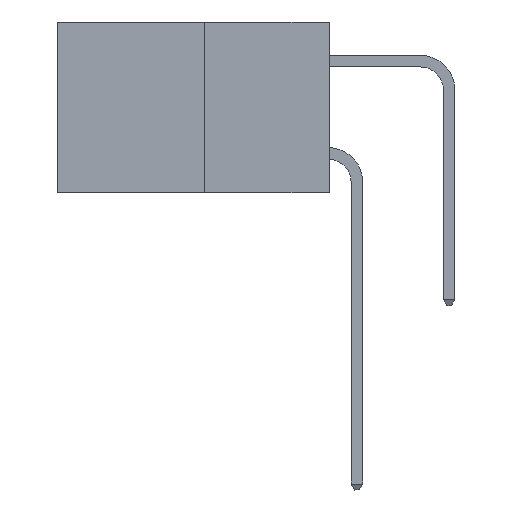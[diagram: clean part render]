
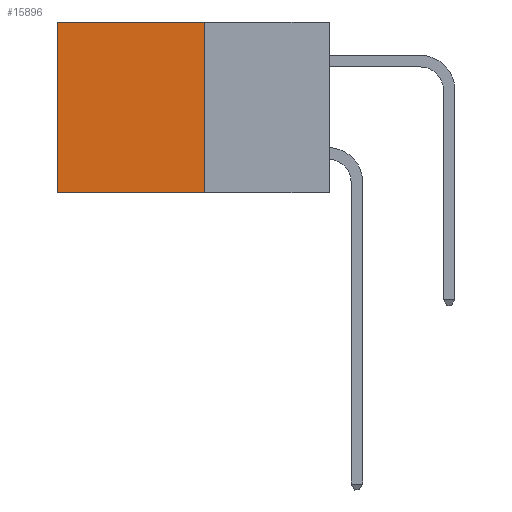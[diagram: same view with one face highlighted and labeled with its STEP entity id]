
A CAD part, left-side view. The second image highlights one B-rep face of the part: STEP entity #15896.
In plain terms, the highlighted planar face has unit normal (-1, 0, 0).
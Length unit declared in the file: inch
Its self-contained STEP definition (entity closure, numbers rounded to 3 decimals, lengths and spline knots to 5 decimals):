
#310 = CARTESIAN_POINT ( 'NONE',  ( 0.277, 0.27, -0.37 ) ) ;
#665 = LINE ( 'NONE', #18422, #26575 ) ;
#683 = FACE_OUTER_BOUND ( 'NONE', #27357, .T. ) ;
#1572 = LINE ( 'NONE', #18201, #24973 ) ;
#1852 = DIRECTION ( 'NONE',  ( 0., 1., 0. ) ) ;
#2089 = DIRECTION ( 'NONE',  ( 0., 0., -1. ) ) ;
#2840 = ORIENTED_EDGE ( 'NONE', *, *, #27835, .T. ) ;
#3052 = VECTOR ( 'NONE', #22208, 39.37008 ) ;
#5921 = CARTESIAN_POINT ( 'NONE',  ( 0.277, 0.59, 0. ) ) ;
#7754 = DIRECTION ( 'NONE',  ( 1., 0., 0. ) ) ;
#8976 = CARTESIAN_POINT ( 'NONE',  ( 0.277, 0.27, -0.37 ) ) ;
#10119 = EDGE_CURVE ( 'NONE', #29624, #12338, #15491, .T. ) ;
#10675 = ORIENTED_EDGE ( 'NONE', *, *, #14356, .T. ) ;
#12098 = LINE ( 'NONE', #27650, #23837 ) ;
#12338 = VERTEX_POINT ( 'NONE', #8976 ) ;
#13613 = EDGE_CURVE ( 'NONE', #12338, #26262, #1572, .T. ) ;
#14356 = EDGE_CURVE ( 'NONE', #29624, #16048, #12098, .T. ) ;
#14727 = CARTESIAN_POINT ( 'NONE',  ( 0.277, 0.27, -0.37 ) ) ;
#15491 = LINE ( 'NONE', #310, #3052 ) ;
#15896 = ADVANCED_FACE ( 'NONE', ( #683 ), #21793, .F. ) ;
#16048 = VERTEX_POINT ( 'NONE', #5921 ) ;
#18201 = CARTESIAN_POINT ( 'NONE',  ( 0.277, 0.27, -0.37 ) ) ;
#18422 = CARTESIAN_POINT ( 'NONE',  ( 0.277, 0.59, -0.37 ) ) ;
#21793 = PLANE ( 'NONE',  #25199 ) ;
#22208 = DIRECTION ( 'NONE',  ( 0., 0., -1. ) ) ;
#22405 = ORIENTED_EDGE ( 'NONE', *, *, #13613, .F. ) ;
#23837 = VECTOR ( 'NONE', #29986, 39.37008 ) ;
#24121 = DIRECTION ( 'NONE',  ( 0., 0., -1. ) ) ;
#24626 = ORIENTED_EDGE ( 'NONE', *, *, #10119, .F. ) ;
#24973 = VECTOR ( 'NONE', #1852, 39.37008 ) ;
#25199 = AXIS2_PLACEMENT_3D ( 'NONE', #14727, #7754, #24121 ) ;
#26055 = CARTESIAN_POINT ( 'NONE',  ( 0.277, 0.27, 0. ) ) ;
#26262 = VERTEX_POINT ( 'NONE', #26992 ) ;
#26575 = VECTOR ( 'NONE', #2089, 39.37008 ) ;
#26992 = CARTESIAN_POINT ( 'NONE',  ( 0.277, 0.59, -0.37 ) ) ;
#27357 = EDGE_LOOP ( 'NONE', ( #2840, #22405, #24626, #10675 ) ) ;
#27650 = CARTESIAN_POINT ( 'NONE',  ( 0.277, 0.27, 0. ) ) ;
#27835 = EDGE_CURVE ( 'NONE', #16048, #26262, #665, .T. ) ;
#29624 = VERTEX_POINT ( 'NONE', #26055 ) ;
#29986 = DIRECTION ( 'NONE',  ( 0., 1., 0. ) ) ;
